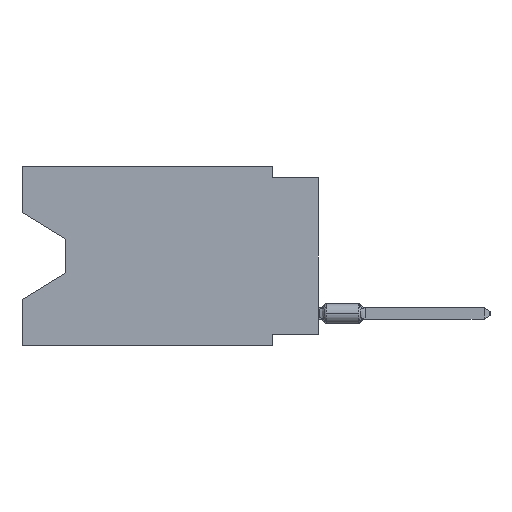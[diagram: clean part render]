
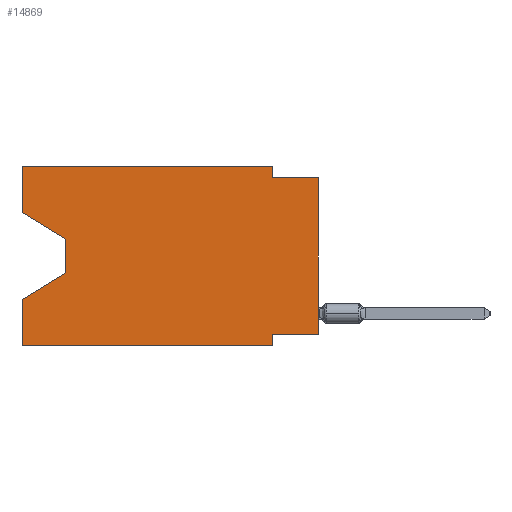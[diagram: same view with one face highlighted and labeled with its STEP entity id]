
A CAD part, left-side view. The second image highlights one B-rep face of the part: STEP entity #14869.
In plain terms, the highlighted planar face has unit normal (-1, 0, 0).
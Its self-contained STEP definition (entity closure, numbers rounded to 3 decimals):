
#328 = LINE ( 'NONE', #63937, #38842 ) ;
#865 = EDGE_CURVE ( 'NONE', #67195, #61631, #65371, .T. ) ;
#899 = VERTEX_POINT ( 'NONE', #71387 ) ;
#1210 = CARTESIAN_POINT ( 'NONE',  ( 0., 2.54, 0. ) ) ;
#2026 = VERTEX_POINT ( 'NONE', #58250 ) ;
#2787 = DIRECTION ( 'NONE',  ( 0., -1., 0. ) ) ;
#2842 = EDGE_CURVE ( 'NONE', #21454, #64702, #30203, .T. ) ;
#3285 = VECTOR ( 'NONE', #58224, 1000. ) ;
#3965 = CARTESIAN_POINT ( 'NONE',  ( 0., 13.97, -5.893 ) ) ;
#4057 = CARTESIAN_POINT ( 'NONE',  ( 0., 2.54, -9.271 ) ) ;
#4111 = VERTEX_POINT ( 'NONE', #22951 ) ;
#5004 = DIRECTION ( 'NONE',  ( 0., -1., 0. ) ) ;
#5851 = EDGE_CURVE ( 'NONE', #61212, #43037, #25105, .T. ) ;
#6074 = CARTESIAN_POINT ( 'NONE',  ( 0., 16.383, 0. ) ) ;
#6102 = CARTESIAN_POINT ( 'NONE',  ( 0., 16.383, 0. ) ) ;
#7242 = EDGE_CURVE ( 'NONE', #43037, #48941, #48366, .T. ) ;
#7409 = EDGE_CURVE ( 'NONE', #41747, #61631, #66751, .T. ) ;
#8542 = CARTESIAN_POINT ( 'NONE',  ( 0., 16.383, 0. ) ) ;
#10921 = ORIENTED_EDGE ( 'NONE', *, *, #27430, .T. ) ;
#12460 = CARTESIAN_POINT ( 'NONE',  ( 0., 0., 0. ) ) ;
#14869 = ADVANCED_FACE ( 'NONE', ( #63673 ), #51317, .F. ) ;
#18105 = LINE ( 'NONE', #12460, #49996 ) ;
#18551 = DIRECTION ( 'NONE',  ( 0., 0.855, -0.519 ) ) ;
#18740 = EDGE_CURVE ( 'NONE', #899, #2026, #49682, .T. ) ;
#19874 = ORIENTED_EDGE ( 'NONE', *, *, #2842, .T. ) ;
#21048 = DIRECTION ( 'NONE',  ( 0., -1., 0. ) ) ;
#21454 = VERTEX_POINT ( 'NONE', #3965 ) ;
#22289 = CARTESIAN_POINT ( 'NONE',  ( 0., 2.54, 0. ) ) ;
#22305 = DIRECTION ( 'NONE',  ( 1., 0., 0. ) ) ;
#22669 = DIRECTION ( 'NONE',  ( 0., 0., -1. ) ) ;
#22951 = CARTESIAN_POINT ( 'NONE',  ( 0., 13.97, -4.013 ) ) ;
#23305 = ORIENTED_EDGE ( 'NONE', *, *, #49506, .T. ) ;
#23956 = EDGE_CURVE ( 'NONE', #56445, #67195, #36747, .T. ) ;
#25105 = LINE ( 'NONE', #8542, #48836 ) ;
#25476 = DIRECTION ( 'NONE',  ( 0., 0., 1. ) ) ;
#27430 = EDGE_CURVE ( 'NONE', #56445, #2026, #18105, .T. ) ;
#27824 = VECTOR ( 'NONE', #58999, 1000. ) ;
#30203 = LINE ( 'NONE', #64825, #71477 ) ;
#30949 = LINE ( 'NONE', #1210, #52340 ) ;
#31478 = CARTESIAN_POINT ( 'NONE',  ( 0., 2.54, -9.906 ) ) ;
#32804 = ORIENTED_EDGE ( 'NONE', *, *, #7242, .F. ) ;
#35635 = CARTESIAN_POINT ( 'NONE',  ( 0., 0., -9.271 ) ) ;
#36225 = DIRECTION ( 'NONE',  ( 0., 0., -1. ) ) ;
#36664 = ORIENTED_EDGE ( 'NONE', *, *, #60195, .F. ) ;
#36747 = LINE ( 'NONE', #35635, #3285 ) ;
#38431 = LINE ( 'NONE', #66314, #47503 ) ;
#38842 = VECTOR ( 'NONE', #69231, 1000. ) ;
#41063 = DIRECTION ( 'NONE',  ( 0., 0., 1. ) ) ;
#41747 = VERTEX_POINT ( 'NONE', #72202 ) ;
#43037 = VERTEX_POINT ( 'NONE', #6074 ) ;
#47015 = ORIENTED_EDGE ( 'NONE', *, *, #865, .F. ) ;
#47503 = VECTOR ( 'NONE', #61039, 1000. ) ;
#47998 = ORIENTED_EDGE ( 'NONE', *, *, #7409, .T. ) ;
#48152 = EDGE_LOOP ( 'NONE', ( #23305, #55904, #19874, #36664, #47998, #47015, #57417, #10921, #71461, #71541, #32804, #73583 ) ) ;
#48366 = LINE ( 'NONE', #60734, #71796 ) ;
#48836 = VECTOR ( 'NONE', #25476, 1000. ) ;
#48941 = VERTEX_POINT ( 'NONE', #22289 ) ;
#49506 = EDGE_CURVE ( 'NONE', #61212, #4111, #328, .T. ) ;
#49682 = LINE ( 'NONE', #72613, #66452 ) ;
#49996 = VECTOR ( 'NONE', #52002, 1000. ) ;
#51317 = PLANE ( 'NONE',  #69619 ) ;
#52002 = DIRECTION ( 'NONE',  ( 0., 0., 1. ) ) ;
#52340 = VECTOR ( 'NONE', #36225, 1000. ) ;
#53499 = CARTESIAN_POINT ( 'NONE',  ( 0., 16.383, 0. ) ) ;
#53850 = EDGE_CURVE ( 'NONE', #48941, #899, #30949, .T. ) ;
#55844 = CARTESIAN_POINT ( 'NONE',  ( 0., 16.383, -9.906 ) ) ;
#55901 = CARTESIAN_POINT ( 'NONE',  ( 0., 16.383, -2.546 ) ) ;
#55904 = ORIENTED_EDGE ( 'NONE', *, *, #69610, .T. ) ;
#56445 = VERTEX_POINT ( 'NONE', #58012 ) ;
#57417 = ORIENTED_EDGE ( 'NONE', *, *, #23956, .F. ) ;
#58012 = CARTESIAN_POINT ( 'NONE',  ( 0., 0., -9.271 ) ) ;
#58224 = DIRECTION ( 'NONE',  ( 0., 1., 0. ) ) ;
#58250 = CARTESIAN_POINT ( 'NONE',  ( 0., 0., -0.635 ) ) ;
#58646 = CARTESIAN_POINT ( 'NONE',  ( 0., 2.54, -9.906 ) ) ;
#58999 = DIRECTION ( 'NONE',  ( 0., 0., -1. ) ) ;
#60195 = EDGE_CURVE ( 'NONE', #41747, #64702, #71151, .T. ) ;
#60734 = CARTESIAN_POINT ( 'NONE',  ( 0., 16.383, 0. ) ) ;
#61039 = DIRECTION ( 'NONE',  ( 0., 0., -1. ) ) ;
#61212 = VERTEX_POINT ( 'NONE', #55901 ) ;
#61631 = VERTEX_POINT ( 'NONE', #58646 ) ;
#62643 = CARTESIAN_POINT ( 'NONE',  ( 0., 16.383, -7.36 ) ) ;
#63673 = FACE_OUTER_BOUND ( 'NONE', #48152, .T. ) ;
#63937 = CARTESIAN_POINT ( 'NONE',  ( 0., 16.383, -2.546 ) ) ;
#64702 = VERTEX_POINT ( 'NONE', #62643 ) ;
#64825 = CARTESIAN_POINT ( 'NONE',  ( 0., 13.97, -5.893 ) ) ;
#65371 = LINE ( 'NONE', #31478, #27824 ) ;
#66314 = CARTESIAN_POINT ( 'NONE',  ( 0., 13.97, -4.013 ) ) ;
#66452 = VECTOR ( 'NONE', #21048, 1000. ) ;
#66751 = LINE ( 'NONE', #55844, #74206 ) ;
#67195 = VERTEX_POINT ( 'NONE', #4057 ) ;
#69231 = DIRECTION ( 'NONE',  ( 0., -0.855, -0.519 ) ) ;
#69610 = EDGE_CURVE ( 'NONE', #4111, #21454, #38431, .T. ) ;
#69619 = AXIS2_PLACEMENT_3D ( 'NONE', #6102, #22305, #22669 ) ;
#69664 = VECTOR ( 'NONE', #41063, 1000. ) ;
#71151 = LINE ( 'NONE', #53499, #69664 ) ;
#71387 = CARTESIAN_POINT ( 'NONE',  ( 0., 2.54, -0.635 ) ) ;
#71461 = ORIENTED_EDGE ( 'NONE', *, *, #18740, .F. ) ;
#71477 = VECTOR ( 'NONE', #18551, 1000. ) ;
#71541 = ORIENTED_EDGE ( 'NONE', *, *, #53850, .F. ) ;
#71796 = VECTOR ( 'NONE', #2787, 1000. ) ;
#72202 = CARTESIAN_POINT ( 'NONE',  ( 0., 16.383, -9.906 ) ) ;
#72613 = CARTESIAN_POINT ( 'NONE',  ( 0., 0., -0.635 ) ) ;
#73583 = ORIENTED_EDGE ( 'NONE', *, *, #5851, .F. ) ;
#74206 = VECTOR ( 'NONE', #5004, 1000. ) ;
